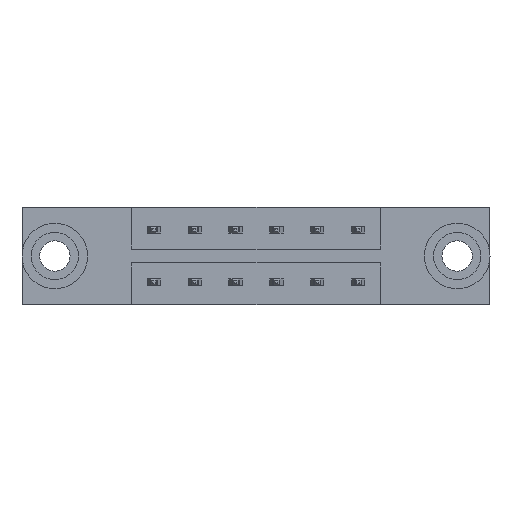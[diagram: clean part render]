
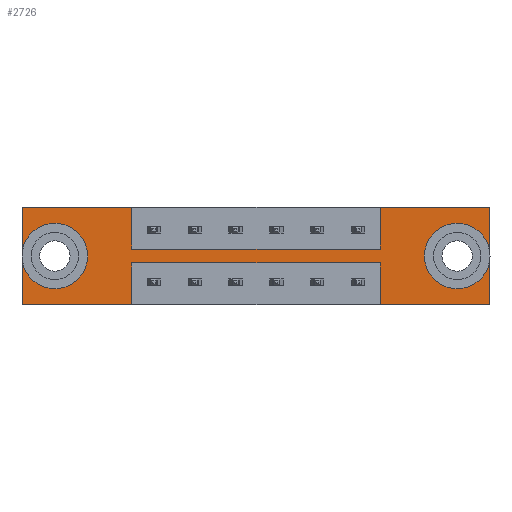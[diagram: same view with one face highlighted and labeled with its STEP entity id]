
A CAD part, front view. The second image highlights one B-rep face of the part: STEP entity #2726.
In plain terms, the highlighted planar face has unit normal (0, -1, 0).
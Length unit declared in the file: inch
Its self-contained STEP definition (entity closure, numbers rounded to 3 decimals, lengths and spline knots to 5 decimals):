
#14 = CARTESIAN_POINT ( 'NONE',  ( 0., 0., -0.37 ) ) ;
#25 = ORIENTED_EDGE ( 'NONE', *, *, #8955, .F. ) ;
#55 = VECTOR ( 'NONE', #2807, 39.37008 ) ;
#180 = VECTOR ( 'NONE', #7264, 39.37008 ) ;
#300 = DIRECTION ( 'NONE',  ( -1., 0., 0. ) ) ;
#491 = DIRECTION ( 'NONE',  ( 0., 0., -1. ) ) ;
#753 = ORIENTED_EDGE ( 'NONE', *, *, #5116, .F. ) ;
#763 = VERTEX_POINT ( 'NONE', #2457 ) ;
#860 = CIRCLE ( 'NONE', #2770, 0.078 ) ;
#873 = CARTESIAN_POINT ( 'NONE',  ( 0., 0., -0.37 ) ) ;
#891 = VERTEX_POINT ( 'NONE', #5977 ) ;
#1066 = EDGE_LOOP ( 'NONE', ( #7445, #25, #2014, #5807, #7656, #4146, #6030, #7872, #2453, #8096, #753, #2697 ) ) ;
#1166 = LINE ( 'NONE', #7287, #4961 ) ;
#1171 = CARTESIAN_POINT ( 'NONE',  ( 1.3665, 0., -0.2115 ) ) ;
#1203 = PLANE ( 'NONE',  #8213 ) ;
#1549 = ORIENTED_EDGE ( 'NONE', *, *, #3262, .T. ) ;
#1729 = VECTOR ( 'NONE', #8431, 39.37008 ) ;
#1732 = VERTEX_POINT ( 'NONE', #4188 ) ;
#1833 = DIRECTION ( 'NONE',  ( 0., 0., -1. ) ) ;
#1842 = FACE_OUTER_BOUND ( 'NONE', #1066, .T. ) ;
#1876 = VECTOR ( 'NONE', #6828, 39.37008 ) ;
#2014 = ORIENTED_EDGE ( 'NONE', *, *, #3415, .F. ) ;
#2043 = LINE ( 'NONE', #9179, #55 ) ;
#2153 = AXIS2_PLACEMENT_3D ( 'NONE', #7469, #3271, #8155 ) ;
#2220 = DIRECTION ( 'NONE',  ( 0., 1., 0. ) ) ;
#2241 = EDGE_CURVE ( 'NONE', #4706, #5708, #8429, .T. ) ;
#2361 = EDGE_CURVE ( 'NONE', #763, #6489, #5955, .T. ) ;
#2453 = ORIENTED_EDGE ( 'NONE', *, *, #2629, .F. ) ;
#2457 = CARTESIAN_POINT ( 'NONE',  ( 1.3665, 0., -0.1585 ) ) ;
#2504 = VERTEX_POINT ( 'NONE', #8951 ) ;
#2544 = VERTEX_POINT ( 'NONE', #7460 ) ;
#2629 = EDGE_CURVE ( 'NONE', #2674, #2544, #2043, .T. ) ;
#2674 = VERTEX_POINT ( 'NONE', #14 ) ;
#2697 = ORIENTED_EDGE ( 'NONE', *, *, #4769, .F. ) ;
#2726 = ADVANCED_FACE ( 'NONE', ( #5419, #8877, #1842 ), #1203, .T. ) ;
#2770 = AXIS2_PLACEMENT_3D ( 'NONE', #6483, #2220, #7168 ) ;
#2781 = EDGE_LOOP ( 'NONE', ( #8809, #1549 ) ) ;
#2807 = DIRECTION ( 'NONE',  ( 0., 0., 1. ) ) ;
#2855 = VECTOR ( 'NONE', #1833, 39.37008 ) ;
#2944 = DIRECTION ( 'NONE',  ( 0., 0., -1. ) ) ;
#2984 = DIRECTION ( 'NONE',  ( 0., 1., 0. ) ) ;
#2991 = CARTESIAN_POINT ( 'NONE',  ( 1.659, 0., -0.185 ) ) ;
#3000 = CIRCLE ( 'NONE', #7812, 0.078 ) ;
#3009 = CARTESIAN_POINT ( 'NONE',  ( 1.659, 0., -0.107 ) ) ;
#3073 = CARTESIAN_POINT ( 'NONE',  ( 0.125, 0., -0.185 ) ) ;
#3077 = VERTEX_POINT ( 'NONE', #4288 ) ;
#3136 = CARTESIAN_POINT ( 'NONE',  ( 0.125, 0., -0.107 ) ) ;
#3147 = EDGE_LOOP ( 'NONE', ( #3486, #9022 ) ) ;
#3262 = EDGE_CURVE ( 'NONE', #6953, #8656, #3000, .T. ) ;
#3271 = DIRECTION ( 'NONE',  ( 0., 1., 0. ) ) ;
#3313 = LINE ( 'NONE', #8022, #6839 ) ;
#3365 = DIRECTION ( 'NONE',  ( 0., 0., -1. ) ) ;
#3415 = EDGE_CURVE ( 'NONE', #6623, #1732, #3655, .T. ) ;
#3463 = DIRECTION ( 'NONE',  ( -1., 0., 0. ) ) ;
#3486 = ORIENTED_EDGE ( 'NONE', *, *, #6414, .T. ) ;
#3544 = VERTEX_POINT ( 'NONE', #6216 ) ;
#3615 = CARTESIAN_POINT ( 'NONE',  ( 0.4175, 0., -0.2115 ) ) ;
#3637 = VECTOR ( 'NONE', #7929, 39.37008 ) ;
#3655 = LINE ( 'NONE', #8843, #1729 ) ;
#3737 = EDGE_CURVE ( 'NONE', #6489, #6623, #1166, .T. ) ;
#3764 = DIRECTION ( 'NONE',  ( 0., 0., 1. ) ) ;
#3815 = LINE ( 'NONE', #8839, #1876 ) ;
#3873 = LINE ( 'NONE', #8610, #3637 ) ;
#3898 = DIRECTION ( 'NONE',  ( 0., 0., 1. ) ) ;
#4128 = VERTEX_POINT ( 'NONE', #3136 ) ;
#4146 = ORIENTED_EDGE ( 'NONE', *, *, #4399, .F. ) ;
#4188 = CARTESIAN_POINT ( 'NONE',  ( 1.784, 0., -0.37 ) ) ;
#4288 = CARTESIAN_POINT ( 'NONE',  ( 0.4175, 0., -0.1585 ) ) ;
#4399 = EDGE_CURVE ( 'NONE', #3077, #763, #3873, .T. ) ;
#4634 = CARTESIAN_POINT ( 'NONE',  ( 1.784, 0., 0. ) ) ;
#4706 = VERTEX_POINT ( 'NONE', #8741 ) ;
#4769 = EDGE_CURVE ( 'NONE', #5708, #6036, #3313, .T. ) ;
#4830 = LINE ( 'NONE', #3615, #6286 ) ;
#4961 = VECTOR ( 'NONE', #7260, 39.37008 ) ;
#5093 = VECTOR ( 'NONE', #300, 39.37008 ) ;
#5116 = EDGE_CURVE ( 'NONE', #6036, #2504, #4830, .T. ) ;
#5419 = FACE_BOUND ( 'NONE', #2781, .T. ) ;
#5480 = DIRECTION ( 'NONE',  ( 0., -1., 0. ) ) ;
#5708 = VERTEX_POINT ( 'NONE', #8660 ) ;
#5782 = LINE ( 'NONE', #8800, #5093 ) ;
#5807 = ORIENTED_EDGE ( 'NONE', *, *, #3737, .F. ) ;
#5955 = LINE ( 'NONE', #7231, #180 ) ;
#5959 = EDGE_CURVE ( 'NONE', #891, #3077, #6593, .T. ) ;
#5977 = CARTESIAN_POINT ( 'NONE',  ( 0.4175, 0., 0. ) ) ;
#6030 = ORIENTED_EDGE ( 'NONE', *, *, #5959, .F. ) ;
#6036 = VERTEX_POINT ( 'NONE', #8949 ) ;
#6108 = EDGE_CURVE ( 'NONE', #2504, #2674, #7782, .T. ) ;
#6156 = CARTESIAN_POINT ( 'NONE',  ( 0.4175, 0., -0.1585 ) ) ;
#6216 = CARTESIAN_POINT ( 'NONE',  ( 0.125, 0., -0.263 ) ) ;
#6286 = VECTOR ( 'NONE', #3365, 39.37008 ) ;
#6414 = EDGE_CURVE ( 'NONE', #4128, #3544, #9040, .T. ) ;
#6470 = CIRCLE ( 'NONE', #2153, 0.078 ) ;
#6483 = CARTESIAN_POINT ( 'NONE',  ( 1.659, 0., -0.185 ) ) ;
#6489 = VERTEX_POINT ( 'NONE', #7317 ) ;
#6593 = LINE ( 'NONE', #6156, #2855 ) ;
#6601 = VECTOR ( 'NONE', #3898, 39.37008 ) ;
#6623 = VERTEX_POINT ( 'NONE', #4634 ) ;
#6828 = DIRECTION ( 'NONE',  ( 1., 0., 0. ) ) ;
#6839 = VECTOR ( 'NONE', #7948, 39.37008 ) ;
#6953 = VERTEX_POINT ( 'NONE', #9089 ) ;
#7168 = DIRECTION ( 'NONE',  ( 0., 0., -1. ) ) ;
#7231 = CARTESIAN_POINT ( 'NONE',  ( 1.3665, 0., -0.1585 ) ) ;
#7260 = DIRECTION ( 'NONE',  ( 1., 0., 0. ) ) ;
#7264 = DIRECTION ( 'NONE',  ( 0., 0., 1. ) ) ;
#7287 = CARTESIAN_POINT ( 'NONE',  ( 0., 0., 0. ) ) ;
#7305 = EDGE_CURVE ( 'NONE', #3544, #4128, #6470, .T. ) ;
#7317 = CARTESIAN_POINT ( 'NONE',  ( 1.3665, 0., 0. ) ) ;
#7346 = VECTOR ( 'NONE', #3463, 39.37008 ) ;
#7445 = ORIENTED_EDGE ( 'NONE', *, *, #2241, .F. ) ;
#7460 = CARTESIAN_POINT ( 'NONE',  ( 0., 0., 0. ) ) ;
#7469 = CARTESIAN_POINT ( 'NONE',  ( 0.125, 0., -0.185 ) ) ;
#7656 = ORIENTED_EDGE ( 'NONE', *, *, #2361, .F. ) ;
#7782 = LINE ( 'NONE', #9011, #7346 ) ;
#7812 = AXIS2_PLACEMENT_3D ( 'NONE', #2991, #2984, #2944 ) ;
#7872 = ORIENTED_EDGE ( 'NONE', *, *, #8184, .F. ) ;
#7929 = DIRECTION ( 'NONE',  ( 1., 0., 0. ) ) ;
#7948 = DIRECTION ( 'NONE',  ( -1., 0., 0. ) ) ;
#7951 = DIRECTION ( 'NONE',  ( 0., 1., 0. ) ) ;
#8022 = CARTESIAN_POINT ( 'NONE',  ( 0.4175, 0., -0.2115 ) ) ;
#8096 = ORIENTED_EDGE ( 'NONE', *, *, #6108, .F. ) ;
#8155 = DIRECTION ( 'NONE',  ( 0., 0., 1. ) ) ;
#8184 = EDGE_CURVE ( 'NONE', #2544, #891, #3815, .T. ) ;
#8213 = AXIS2_PLACEMENT_3D ( 'NONE', #873, #5480, #491 ) ;
#8429 = LINE ( 'NONE', #1171, #6601 ) ;
#8431 = DIRECTION ( 'NONE',  ( 0., 0., -1. ) ) ;
#8595 = EDGE_CURVE ( 'NONE', #8656, #6953, #860, .T. ) ;
#8610 = CARTESIAN_POINT ( 'NONE',  ( 0.4175, 0., -0.1585 ) ) ;
#8656 = VERTEX_POINT ( 'NONE', #3009 ) ;
#8660 = CARTESIAN_POINT ( 'NONE',  ( 1.3665, 0., -0.2115 ) ) ;
#8741 = CARTESIAN_POINT ( 'NONE',  ( 1.3665, 0., -0.37 ) ) ;
#8800 = CARTESIAN_POINT ( 'NONE',  ( 0., 0., -0.37 ) ) ;
#8809 = ORIENTED_EDGE ( 'NONE', *, *, #8595, .T. ) ;
#8839 = CARTESIAN_POINT ( 'NONE',  ( 0., 0., 0. ) ) ;
#8843 = CARTESIAN_POINT ( 'NONE',  ( 1.784, 0., 0. ) ) ;
#8877 = FACE_BOUND ( 'NONE', #3147, .T. ) ;
#8949 = CARTESIAN_POINT ( 'NONE',  ( 0.4175, 0., -0.2115 ) ) ;
#8951 = CARTESIAN_POINT ( 'NONE',  ( 0.4175, 0., -0.37 ) ) ;
#8955 = EDGE_CURVE ( 'NONE', #1732, #4706, #5782, .T. ) ;
#9011 = CARTESIAN_POINT ( 'NONE',  ( 0., 0., -0.37 ) ) ;
#9022 = ORIENTED_EDGE ( 'NONE', *, *, #7305, .T. ) ;
#9040 = CIRCLE ( 'NONE', #9057, 0.078 ) ;
#9057 = AXIS2_PLACEMENT_3D ( 'NONE', #3073, #7951, #3764 ) ;
#9089 = CARTESIAN_POINT ( 'NONE',  ( 1.659, 0., -0.263 ) ) ;
#9179 = CARTESIAN_POINT ( 'NONE',  ( 0., 0., 0. ) ) ;
